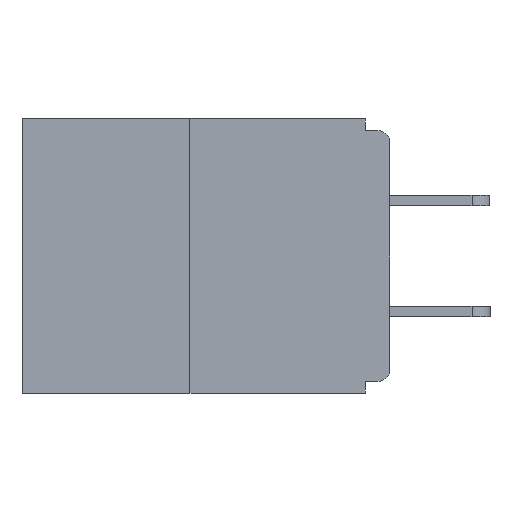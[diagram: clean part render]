
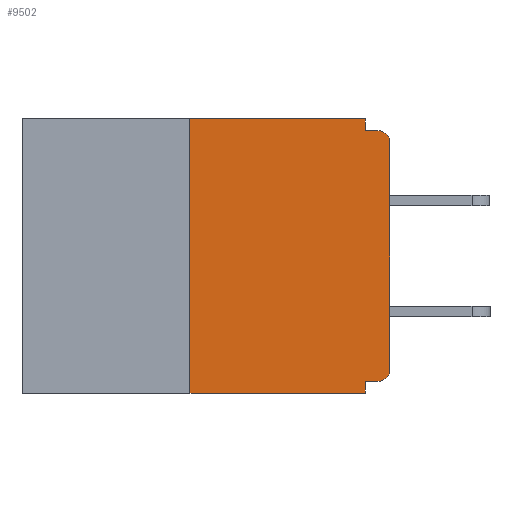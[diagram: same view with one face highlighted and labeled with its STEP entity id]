
A CAD part, left-side view. The second image highlights one B-rep face of the part: STEP entity #9502.
In plain terms, the highlighted planar face has unit normal (-1, 0, 0).
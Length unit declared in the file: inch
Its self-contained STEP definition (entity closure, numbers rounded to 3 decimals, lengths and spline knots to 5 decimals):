
#239 = VECTOR ( 'NONE', #10024, 39.37008 ) ;
#577 = LINE ( 'NONE', #5457, #17906 ) ;
#905 = VECTOR ( 'NONE', #4204, 39.37008 ) ;
#1861 = ORIENTED_EDGE ( 'NONE', *, *, #16579, .T. ) ;
#2154 = CARTESIAN_POINT ( 'NONE',  ( 0., 0., 0. ) ) ;
#2724 = VECTOR ( 'NONE', #9047, 39.37008 ) ;
#2785 = VERTEX_POINT ( 'NONE', #13750 ) ;
#3502 = VERTEX_POINT ( 'NONE', #14169 ) ;
#3504 = LINE ( 'NONE', #2154, #2724 ) ;
#3563 = CARTESIAN_POINT ( 'NONE',  ( 0., 0.031, -0.015 ) ) ;
#3629 = ORIENTED_EDGE ( 'NONE', *, *, #9875, .F. ) ;
#3690 = CARTESIAN_POINT ( 'NONE',  ( 0., 0.031, -0.343 ) ) ;
#3761 = DIRECTION ( 'NONE',  ( 0., -1., 0. ) ) ;
#4041 = CARTESIAN_POINT ( 'NONE',  ( 0., 0.25, 0. ) ) ;
#4158 = PLANE ( 'NONE',  #15544 ) ;
#4204 = DIRECTION ( 'NONE',  ( 0., 1., 0. ) ) ;
#4288 = LINE ( 'NONE', #9184, #905 ) ;
#4524 = VECTOR ( 'NONE', #7091, 39.37008 ) ;
#4958 = DIRECTION ( 'NONE',  ( -1., 0., 0. ) ) ;
#5457 = CARTESIAN_POINT ( 'NONE',  ( 0., 0.031, 0. ) ) ;
#6021 = CIRCLE ( 'NONE', #11449, 0.015 ) ;
#6379 = CARTESIAN_POINT ( 'NONE',  ( 0., 0.25, 0. ) ) ;
#6634 = EDGE_CURVE ( 'NONE', #2785, #13769, #3504, .T. ) ;
#6873 = EDGE_CURVE ( 'NONE', #16209, #8789, #4288, .T. ) ;
#7021 = CARTESIAN_POINT ( 'NONE',  ( 0., 0.46, -0.343 ) ) ;
#7091 = DIRECTION ( 'NONE',  ( 0., 0., -1. ) ) ;
#7637 = CARTESIAN_POINT ( 'NONE',  ( 0., 0.015, -0.328 ) ) ;
#7859 = VERTEX_POINT ( 'NONE', #14103 ) ;
#8189 = LINE ( 'NONE', #13597, #12932 ) ;
#8447 = LINE ( 'NONE', #3690, #4524 ) ;
#8460 = DIRECTION ( 'NONE',  ( 0., -1., 0. ) ) ;
#8462 = EDGE_CURVE ( 'NONE', #3502, #21737, #577, .T. ) ;
#8606 = ORIENTED_EDGE ( 'NONE', *, *, #8462, .F. ) ;
#8789 = VERTEX_POINT ( 'NONE', #13072 ) ;
#8979 = DIRECTION ( 'NONE',  ( 0., 0., -1. ) ) ;
#9047 = DIRECTION ( 'NONE',  ( 0., 0., 1. ) ) ;
#9184 = CARTESIAN_POINT ( 'NONE',  ( 0., 0., -0.328 ) ) ;
#9502 = ADVANCED_FACE ( 'NONE', ( #18939 ), #4158, .F. ) ;
#9875 = EDGE_CURVE ( 'NONE', #7859, #17533, #14932, .T. ) ;
#9895 = EDGE_CURVE ( 'NONE', #16209, #2785, #6021, .T. ) ;
#10024 = DIRECTION ( 'NONE',  ( 0., 0., 1. ) ) ;
#10207 = VERTEX_POINT ( 'NONE', #12737 ) ;
#10562 = LINE ( 'NONE', #7021, #15034 ) ;
#10757 = VECTOR ( 'NONE', #21276, 39.37008 ) ;
#10960 = ORIENTED_EDGE ( 'NONE', *, *, #6873, .F. ) ;
#11449 = AXIS2_PLACEMENT_3D ( 'NONE', #18270, #4958, #15079 ) ;
#11668 = EDGE_CURVE ( 'NONE', #21737, #12523, #20778, .T. ) ;
#12132 = EDGE_LOOP ( 'NONE', ( #14815, #3629, #1861, #13570, #10960, #16680, #16482, #16781, #20608, #8606 ) ) ;
#12443 = DIRECTION ( 'NONE',  ( 0., 0., -1. ) ) ;
#12523 = VERTEX_POINT ( 'NONE', #15851 ) ;
#12737 = CARTESIAN_POINT ( 'NONE',  ( 0., 0.031, -0.343 ) ) ;
#12932 = VECTOR ( 'NONE', #8460, 39.37008 ) ;
#13072 = CARTESIAN_POINT ( 'NONE',  ( 0., 0.031, -0.328 ) ) ;
#13570 = ORIENTED_EDGE ( 'NONE', *, *, #20285, .F. ) ;
#13597 = CARTESIAN_POINT ( 'NONE',  ( 0., 0.46, 0. ) ) ;
#13750 = CARTESIAN_POINT ( 'NONE',  ( 0., 0., -0.313 ) ) ;
#13769 = VERTEX_POINT ( 'NONE', #14419 ) ;
#14103 = CARTESIAN_POINT ( 'NONE',  ( 0., 0.25, -0.343 ) ) ;
#14126 = DIRECTION ( 'NONE',  ( 0., 0., -1. ) ) ;
#14169 = CARTESIAN_POINT ( 'NONE',  ( 0., 0.031, 0. ) ) ;
#14419 = CARTESIAN_POINT ( 'NONE',  ( 0., 0., -0.03 ) ) ;
#14815 = ORIENTED_EDGE ( 'NONE', *, *, #20283, .F. ) ;
#14932 = LINE ( 'NONE', #6379, #239 ) ;
#15034 = VECTOR ( 'NONE', #3761, 39.37008 ) ;
#15079 = DIRECTION ( 'NONE',  ( 0., 0., -1. ) ) ;
#15325 = CIRCLE ( 'NONE', #16608, 0.015 ) ;
#15544 = AXIS2_PLACEMENT_3D ( 'NONE', #15815, #17756, #12443 ) ;
#15662 = EDGE_CURVE ( 'NONE', #13769, #12523, #15325, .T. ) ;
#15815 = CARTESIAN_POINT ( 'NONE',  ( 0., 0.46, 0. ) ) ;
#15851 = CARTESIAN_POINT ( 'NONE',  ( 0., 0.015, -0.015 ) ) ;
#15883 = DIRECTION ( 'NONE',  ( -1., 0., 0. ) ) ;
#16209 = VERTEX_POINT ( 'NONE', #7637 ) ;
#16482 = ORIENTED_EDGE ( 'NONE', *, *, #6634, .T. ) ;
#16579 = EDGE_CURVE ( 'NONE', #7859, #10207, #10562, .T. ) ;
#16608 = AXIS2_PLACEMENT_3D ( 'NONE', #19207, #15883, #14126 ) ;
#16680 = ORIENTED_EDGE ( 'NONE', *, *, #9895, .T. ) ;
#16781 = ORIENTED_EDGE ( 'NONE', *, *, #15662, .T. ) ;
#17533 = VERTEX_POINT ( 'NONE', #4041 ) ;
#17756 = DIRECTION ( 'NONE',  ( 1., 0., 0. ) ) ;
#17906 = VECTOR ( 'NONE', #8979, 39.37008 ) ;
#18270 = CARTESIAN_POINT ( 'NONE',  ( 0., 0.015, -0.313 ) ) ;
#18939 = FACE_OUTER_BOUND ( 'NONE', #12132, .T. ) ;
#19207 = CARTESIAN_POINT ( 'NONE',  ( 0., 0.015, -0.03 ) ) ;
#19576 = CARTESIAN_POINT ( 'NONE',  ( 0., 0., -0.015 ) ) ;
#20283 = EDGE_CURVE ( 'NONE', #17533, #3502, #8189, .T. ) ;
#20285 = EDGE_CURVE ( 'NONE', #8789, #10207, #8447, .T. ) ;
#20608 = ORIENTED_EDGE ( 'NONE', *, *, #11668, .F. ) ;
#20778 = LINE ( 'NONE', #19576, #10757 ) ;
#21276 = DIRECTION ( 'NONE',  ( 0., -1., 0. ) ) ;
#21737 = VERTEX_POINT ( 'NONE', #3563 ) ;
